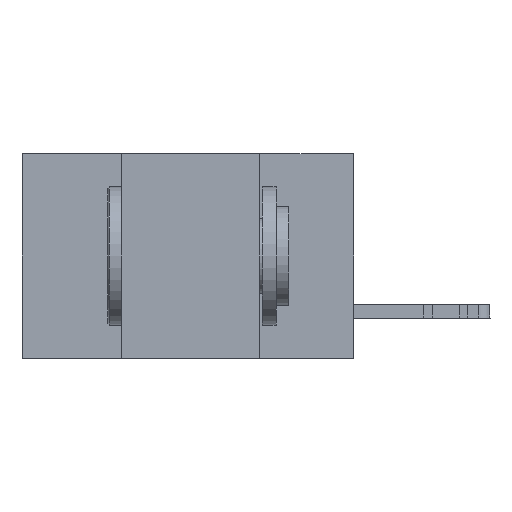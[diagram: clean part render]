
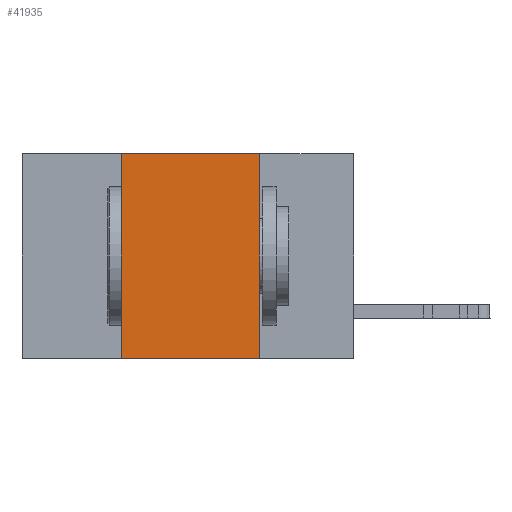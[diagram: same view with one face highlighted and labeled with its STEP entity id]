
A CAD part, left-side view. The second image highlights one B-rep face of the part: STEP entity #41935.
In plain terms, the highlighted planar face has unit normal (-1, 0, 0).
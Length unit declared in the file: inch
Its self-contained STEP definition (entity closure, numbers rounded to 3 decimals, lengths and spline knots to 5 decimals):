
#1607 = CARTESIAN_POINT ( 'NONE',  ( 0., 0.17, 0. ) ) ;
#2084 = LINE ( 'NONE', #12278, #4212 ) ;
#2813 = DIRECTION ( 'NONE',  ( 0., 0., -1. ) ) ;
#3335 = AXIS2_PLACEMENT_3D ( 'NONE', #31359, #17996, #11949 ) ;
#4212 = VECTOR ( 'NONE', #35472, 39.37008 ) ;
#5684 = CARTESIAN_POINT ( 'NONE',  ( 0., 0.6, -0.37 ) ) ;
#7217 = ORIENTED_EDGE ( 'NONE', *, *, #14811, .F. ) ;
#7850 = PLANE ( 'NONE',  #3335 ) ;
#8343 = LINE ( 'NONE', #32362, #40821 ) ;
#11015 = VERTEX_POINT ( 'NONE', #41753 ) ;
#11949 = DIRECTION ( 'NONE',  ( 0., 0., -1. ) ) ;
#12219 = DIRECTION ( 'NONE',  ( 0., -1., 0. ) ) ;
#12278 = CARTESIAN_POINT ( 'NONE',  ( 0., 0.42, 0. ) ) ;
#12656 = VECTOR ( 'NONE', #2813, 39.37008 ) ;
#14087 = EDGE_LOOP ( 'NONE', ( #18378, #31519, #7217, #19783 ) ) ;
#14811 = EDGE_CURVE ( 'NONE', #11015, #22252, #2084, .T. ) ;
#16619 = CARTESIAN_POINT ( 'NONE',  ( 0., 0.42, 0. ) ) ;
#17996 = DIRECTION ( 'NONE',  ( 1., 0., 0. ) ) ;
#18378 = ORIENTED_EDGE ( 'NONE', *, *, #43409, .F. ) ;
#18644 = CARTESIAN_POINT ( 'NONE',  ( 0., 0.17, -0.37 ) ) ;
#19783 = ORIENTED_EDGE ( 'NONE', *, *, #21220, .T. ) ;
#20580 = VERTEX_POINT ( 'NONE', #1607 ) ;
#21220 = EDGE_CURVE ( 'NONE', #11015, #40296, #30754, .T. ) ;
#22252 = VERTEX_POINT ( 'NONE', #16619 ) ;
#22990 = CARTESIAN_POINT ( 'NONE',  ( 0., 0.17, 0. ) ) ;
#25356 = FACE_OUTER_BOUND ( 'NONE', #14087, .T. ) ;
#30754 = LINE ( 'NONE', #5684, #32876 ) ;
#31359 = CARTESIAN_POINT ( 'NONE',  ( 0., 0.6, 0. ) ) ;
#31519 = ORIENTED_EDGE ( 'NONE', *, *, #37910, .F. ) ;
#31588 = LINE ( 'NONE', #22990, #12656 ) ;
#32362 = CARTESIAN_POINT ( 'NONE',  ( 0., 0.6, 0. ) ) ;
#32876 = VECTOR ( 'NONE', #35627, 39.37008 ) ;
#35472 = DIRECTION ( 'NONE',  ( 0., 0., 1. ) ) ;
#35627 = DIRECTION ( 'NONE',  ( 0., -1., 0. ) ) ;
#37910 = EDGE_CURVE ( 'NONE', #22252, #20580, #8343, .T. ) ;
#40296 = VERTEX_POINT ( 'NONE', #18644 ) ;
#40821 = VECTOR ( 'NONE', #12219, 39.37008 ) ;
#41753 = CARTESIAN_POINT ( 'NONE',  ( 0., 0.42, -0.37 ) ) ;
#41935 = ADVANCED_FACE ( 'NONE', ( #25356 ), #7850, .F. ) ;
#43409 = EDGE_CURVE ( 'NONE', #20580, #40296, #31588, .T. ) ;
